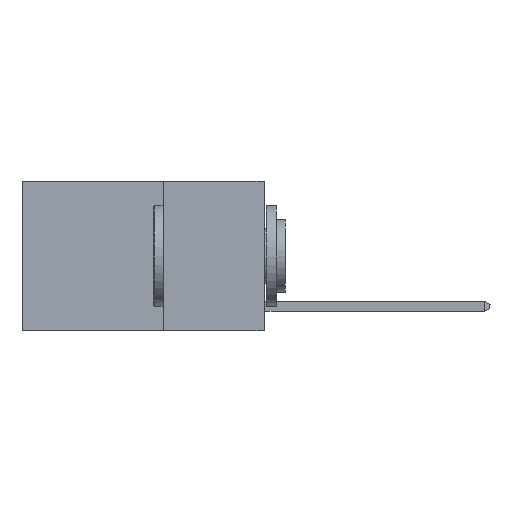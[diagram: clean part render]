
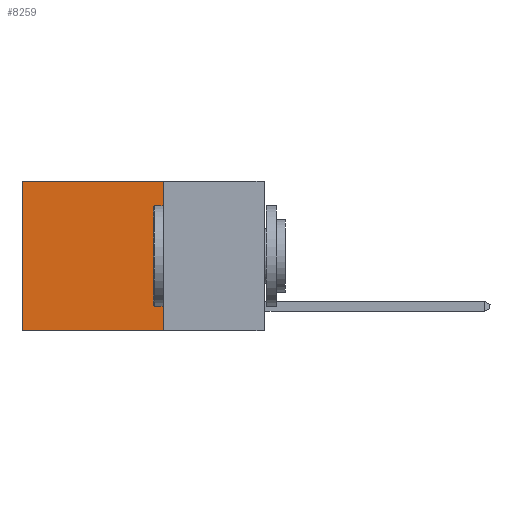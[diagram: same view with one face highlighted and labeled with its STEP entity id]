
A CAD part, left-side view. The second image highlights one B-rep face of the part: STEP entity #8259.
In plain terms, the highlighted planar face has unit normal (-1, 0, 0).
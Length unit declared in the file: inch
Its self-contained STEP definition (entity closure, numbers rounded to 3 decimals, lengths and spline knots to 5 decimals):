
#1458 = VECTOR ( 'NONE', #19841, 39.37008 ) ;
#1633 = DIRECTION ( 'NONE',  ( 0., 0., -1. ) ) ;
#1851 = VERTEX_POINT ( 'NONE', #3370 ) ;
#2657 = CARTESIAN_POINT ( 'NONE',  ( 0.2625, 0.6, 0. ) ) ;
#3238 = VECTOR ( 'NONE', #11819, 39.37008 ) ;
#3370 = CARTESIAN_POINT ( 'NONE',  ( 0.2625, 0.25, 0. ) ) ;
#3702 = VECTOR ( 'NONE', #9575, 39.37008 ) ;
#4625 = LINE ( 'NONE', #18849, #3702 ) ;
#5548 = CARTESIAN_POINT ( 'NONE',  ( 0.2625, 0.25, 0. ) ) ;
#6188 = CARTESIAN_POINT ( 'NONE',  ( 0.2625, 0.25, -0.37 ) ) ;
#6191 = ORIENTED_EDGE ( 'NONE', *, *, #22621, .T. ) ;
#6711 = VERTEX_POINT ( 'NONE', #19174 ) ;
#8259 = ADVANCED_FACE ( 'NONE', ( #17962 ), #12862, .F. ) ;
#8618 = LINE ( 'NONE', #6188, #1458 ) ;
#9575 = DIRECTION ( 'NONE',  ( 0., 1., 0. ) ) ;
#9745 = EDGE_CURVE ( 'NONE', #1851, #6711, #4625, .T. ) ;
#10945 = CARTESIAN_POINT ( 'NONE',  ( 0.2625, 0.25, 0. ) ) ;
#11614 = VECTOR ( 'NONE', #25965, 39.37008 ) ;
#11819 = DIRECTION ( 'NONE',  ( 0., 0., -1. ) ) ;
#12862 = PLANE ( 'NONE',  #17534 ) ;
#14892 = EDGE_CURVE ( 'NONE', #14896, #17609, #8618, .T. ) ;
#14896 = VERTEX_POINT ( 'NONE', #22249 ) ;
#17534 = AXIS2_PLACEMENT_3D ( 'NONE', #10945, #22176, #1633 ) ;
#17609 = VERTEX_POINT ( 'NONE', #24037 ) ;
#17962 = FACE_OUTER_BOUND ( 'NONE', #29072, .T. ) ;
#18849 = CARTESIAN_POINT ( 'NONE',  ( 0.2625, 0.25, 0. ) ) ;
#19174 = CARTESIAN_POINT ( 'NONE',  ( 0.2625, 0.6, 0. ) ) ;
#19338 = LINE ( 'NONE', #5548, #11614 ) ;
#19841 = DIRECTION ( 'NONE',  ( 0., 1., 0. ) ) ;
#22176 = DIRECTION ( 'NONE',  ( 1., 0., 0. ) ) ;
#22249 = CARTESIAN_POINT ( 'NONE',  ( 0.2625, 0.25, -0.37 ) ) ;
#22621 = EDGE_CURVE ( 'NONE', #6711, #17609, #23211, .T. ) ;
#23211 = LINE ( 'NONE', #2657, #3238 ) ;
#24037 = CARTESIAN_POINT ( 'NONE',  ( 0.2625, 0.6, -0.37 ) ) ;
#24133 = ORIENTED_EDGE ( 'NONE', *, *, #28470, .F. ) ;
#25965 = DIRECTION ( 'NONE',  ( 0., 0., -1. ) ) ;
#27738 = ORIENTED_EDGE ( 'NONE', *, *, #9745, .T. ) ;
#28470 = EDGE_CURVE ( 'NONE', #1851, #14896, #19338, .T. ) ;
#29072 = EDGE_LOOP ( 'NONE', ( #6191, #29134, #24133, #27738 ) ) ;
#29134 = ORIENTED_EDGE ( 'NONE', *, *, #14892, .F. ) ;
